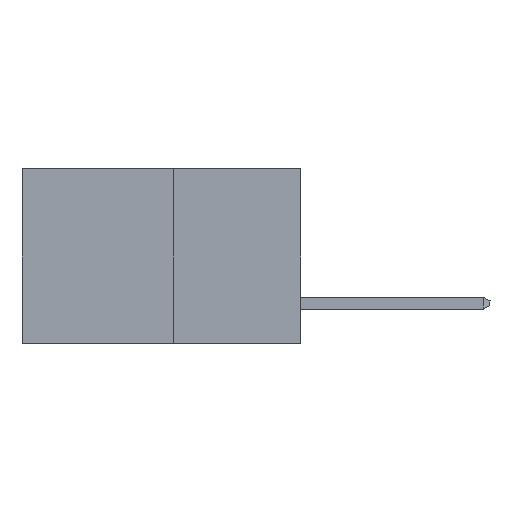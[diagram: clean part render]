
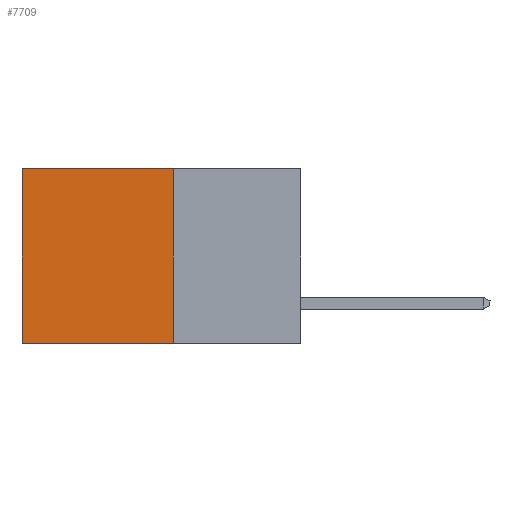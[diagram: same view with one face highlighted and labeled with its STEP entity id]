
A CAD part, left-side view. The second image highlights one B-rep face of the part: STEP entity #7709.
In plain terms, the highlighted planar face has unit normal (-1, 0, 0).
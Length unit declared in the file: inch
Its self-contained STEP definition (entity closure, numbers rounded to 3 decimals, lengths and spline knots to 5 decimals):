
#757 = ORIENTED_EDGE ( 'NONE', *, *, #7356, .T. ) ;
#856 = ORIENTED_EDGE ( 'NONE', *, *, #17974, .F. ) ;
#865 = CARTESIAN_POINT ( 'NONE',  ( 0.277, 0.59, -0.37 ) ) ;
#887 = VERTEX_POINT ( 'NONE', #865 ) ;
#1337 = LINE ( 'NONE', #6025, #8942 ) ;
#1531 = DIRECTION ( 'NONE',  ( 0., 1., 0. ) ) ;
#2911 = FACE_OUTER_BOUND ( 'NONE', #26842, .T. ) ;
#3002 = DIRECTION ( 'NONE',  ( 0., 0., -1. ) ) ;
#3028 = CARTESIAN_POINT ( 'NONE',  ( 0.277, 0.27, -0.37 ) ) ;
#5454 = EDGE_CURVE ( 'NONE', #23966, #12169, #21426, .T. ) ;
#6020 = LINE ( 'NONE', #3028, #26365 ) ;
#6025 = CARTESIAN_POINT ( 'NONE',  ( 0.277, 0.59, -0.37 ) ) ;
#7356 = EDGE_CURVE ( 'NONE', #12169, #887, #1337, .T. ) ;
#7709 = ADVANCED_FACE ( 'NONE', ( #2911 ), #32835, .F. ) ;
#8691 = LINE ( 'NONE', #20828, #28197 ) ;
#8942 = VECTOR ( 'NONE', #31531, 39.37008 ) ;
#12169 = VERTEX_POINT ( 'NONE', #21231 ) ;
#12620 = DIRECTION ( 'NONE',  ( 1., 0., 0. ) ) ;
#13638 = AXIS2_PLACEMENT_3D ( 'NONE', #27826, #12620, #30386 ) ;
#15452 = VECTOR ( 'NONE', #1531, 39.37008 ) ;
#15468 = EDGE_CURVE ( 'NONE', #23966, #18253, #8691, .T. ) ;
#17974 = EDGE_CURVE ( 'NONE', #18253, #887, #6020, .T. ) ;
#18019 = ORIENTED_EDGE ( 'NONE', *, *, #15468, .F. ) ;
#18253 = VERTEX_POINT ( 'NONE', #32083 ) ;
#20828 = CARTESIAN_POINT ( 'NONE',  ( 0.277, 0.27, -0.37 ) ) ;
#21231 = CARTESIAN_POINT ( 'NONE',  ( 0.277, 0.59, 0. ) ) ;
#21426 = LINE ( 'NONE', #29483, #15452 ) ;
#23897 = CARTESIAN_POINT ( 'NONE',  ( 0.277, 0.27, 0. ) ) ;
#23966 = VERTEX_POINT ( 'NONE', #23897 ) ;
#24063 = ORIENTED_EDGE ( 'NONE', *, *, #5454, .T. ) ;
#26365 = VECTOR ( 'NONE', #28412, 39.37008 ) ;
#26842 = EDGE_LOOP ( 'NONE', ( #757, #856, #18019, #24063 ) ) ;
#27826 = CARTESIAN_POINT ( 'NONE',  ( 0.277, 0.27, -0.37 ) ) ;
#28197 = VECTOR ( 'NONE', #3002, 39.37008 ) ;
#28412 = DIRECTION ( 'NONE',  ( 0., 1., 0. ) ) ;
#29483 = CARTESIAN_POINT ( 'NONE',  ( 0.277, 0.27, 0. ) ) ;
#30386 = DIRECTION ( 'NONE',  ( 0., 0., -1. ) ) ;
#31531 = DIRECTION ( 'NONE',  ( 0., 0., -1. ) ) ;
#32083 = CARTESIAN_POINT ( 'NONE',  ( 0.277, 0.27, -0.37 ) ) ;
#32835 = PLANE ( 'NONE',  #13638 ) ;
